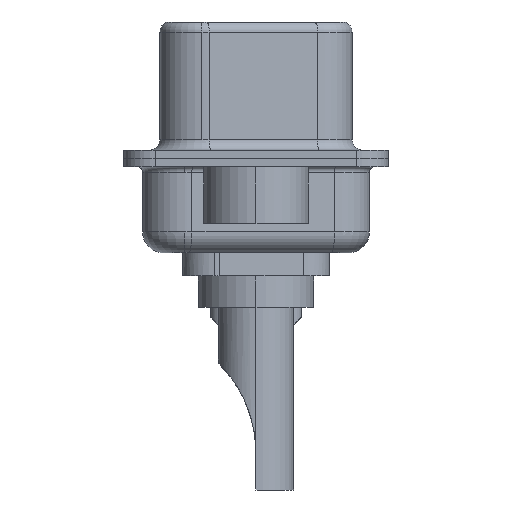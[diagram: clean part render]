
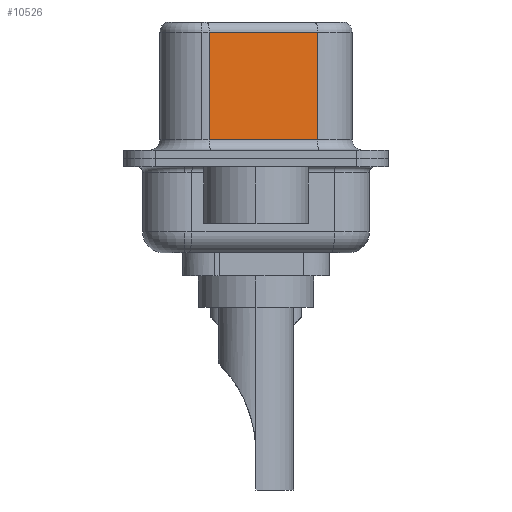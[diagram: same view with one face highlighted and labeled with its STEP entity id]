
A CAD part, left-side view. The second image highlights one B-rep face of the part: STEP entity #10526.
In plain terms, the highlighted planar face has unit normal (-0.985, -0.174, 0).
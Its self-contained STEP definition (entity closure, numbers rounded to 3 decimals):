
#1186 = LINE ( 'NONE', #5537, #16014 ) ;
#1451 = CARTESIAN_POINT ( 'NONE',  ( 4.585, -2.927, 0.9 ) ) ;
#1727 = DIRECTION ( 'NONE',  ( 0., 0., -1. ) ) ;
#1945 = VECTOR ( 'NONE', #5925, 1000. ) ;
#2527 = VECTOR ( 'NONE', #5625, 1000. ) ;
#4164 = AXIS2_PLACEMENT_3D ( 'NONE', #4527, #17342, #8920 ) ;
#4527 = CARTESIAN_POINT ( 'NONE',  ( 4.585, -2.927, 6.52 ) ) ;
#4999 = FACE_OUTER_BOUND ( 'NONE', #11092, .T. ) ;
#5537 = CARTESIAN_POINT ( 'NONE',  ( 4.585, -2.927, 6.02 ) ) ;
#5543 = ORIENTED_EDGE ( 'NONE', *, *, #13234, .F. ) ;
#5625 = DIRECTION ( 'NONE',  ( 0., 0., -1. ) ) ;
#5790 = VERTEX_POINT ( 'NONE', #15375 ) ;
#5925 = DIRECTION ( 'NONE',  ( 0.174, -0.985, 0. ) ) ;
#6244 = VERTEX_POINT ( 'NONE', #12818 ) ;
#6389 = VERTEX_POINT ( 'NONE', #18274 ) ;
#6654 = CARTESIAN_POINT ( 'NONE',  ( 3.675, 2.233, 0.9 ) ) ;
#7543 = PLANE ( 'NONE',  #4164 ) ;
#7745 = CARTESIAN_POINT ( 'NONE',  ( 3.675, 2.233, 6.52 ) ) ;
#8268 = EDGE_CURVE ( 'NONE', #6244, #8414, #14931, .T. ) ;
#8414 = VERTEX_POINT ( 'NONE', #6654 ) ;
#8536 = ORIENTED_EDGE ( 'NONE', *, *, #8268, .T. ) ;
#8920 = DIRECTION ( 'NONE',  ( -0.174, 0.985, 0. ) ) ;
#10466 = EDGE_CURVE ( 'NONE', #8414, #5790, #13378, .T. ) ;
#10526 = ADVANCED_FACE ( 'NONE', ( #4999 ), #7543, .F. ) ;
#11092 = EDGE_LOOP ( 'NONE', ( #5543, #14877, #8536, #16497 ) ) ;
#12214 = EDGE_CURVE ( 'NONE', #6389, #6244, #1186, .T. ) ;
#12818 = CARTESIAN_POINT ( 'NONE',  ( 3.675, 2.233, 6.02 ) ) ;
#13234 = EDGE_CURVE ( 'NONE', #6389, #5790, #17349, .T. ) ;
#13378 = LINE ( 'NONE', #1451, #1945 ) ;
#14877 = ORIENTED_EDGE ( 'NONE', *, *, #12214, .T. ) ;
#14931 = LINE ( 'NONE', #7745, #18351 ) ;
#15335 = DIRECTION ( 'NONE',  ( -0.174, 0.985, 0. ) ) ;
#15375 = CARTESIAN_POINT ( 'NONE',  ( 4.585, -2.927, 0.9 ) ) ;
#16014 = VECTOR ( 'NONE', #15335, 1000. ) ;
#16497 = ORIENTED_EDGE ( 'NONE', *, *, #10466, .T. ) ;
#17342 = DIRECTION ( 'NONE',  ( 0.985, 0.174, 0. ) ) ;
#17349 = LINE ( 'NONE', #18280, #2527 ) ;
#18274 = CARTESIAN_POINT ( 'NONE',  ( 4.585, -2.927, 6.02 ) ) ;
#18280 = CARTESIAN_POINT ( 'NONE',  ( 4.585, -2.927, 6.52 ) ) ;
#18351 = VECTOR ( 'NONE', #1727, 1000. ) ;
